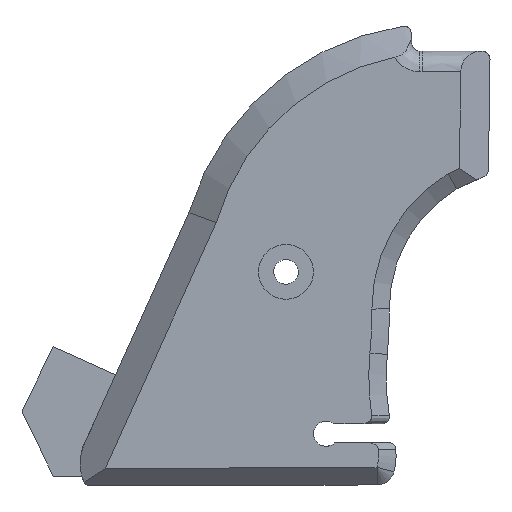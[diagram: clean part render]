
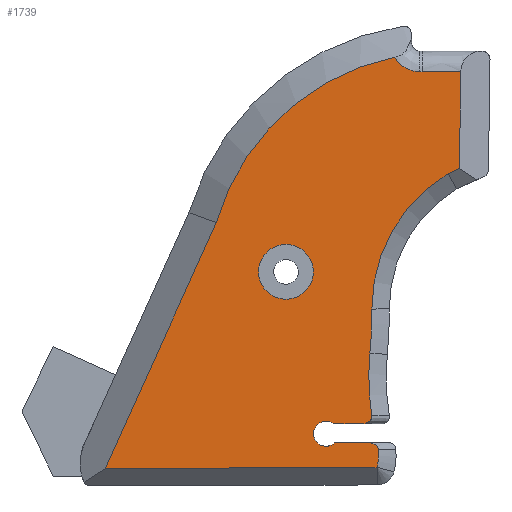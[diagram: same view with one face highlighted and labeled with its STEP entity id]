
A CAD part, left-side view. The second image highlights one B-rep face of the part: STEP entity #1739.
In plain terms, the highlighted planar face has unit normal (-1, 0, 0).
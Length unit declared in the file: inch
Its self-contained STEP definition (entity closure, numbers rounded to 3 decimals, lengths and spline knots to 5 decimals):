
#44=FACE_BOUND('',#590,.T.);
#51=PLANE('',#1873);
#114=CIRCLE('',#1874,0.08642);
#115=CIRCLE('',#1875,1.78527);
#116=CIRCLE('',#1876,3.16162);
#117=CIRCLE('',#1877,1.08448);
#118=CIRCLE('',#1878,1.6175);
#119=CIRCLE('',#1879,0.00059);
#120=CIRCLE('',#1880,0.36222);
#121=CIRCLE('',#1881,0.18906);
#183=LINE('',#2847,#329);
#184=LINE('',#2851,#330);
#185=LINE('',#2872,#331);
#186=LINE('',#2874,#332);
#187=LINE('',#2894,#333);
#188=LINE('',#2896,#334);
#329=VECTOR('',#2102,0.3937);
#330=VECTOR('',#2105,0.3937);
#331=VECTOR('',#2112,0.3937);
#332=VECTOR('',#2113,0.3937);
#333=VECTOR('',#2116,0.3937);
#334=VECTOR('',#2117,0.3937);
#490=FACE_OUTER_BOUND('',#589,.T.);
#589=EDGE_LOOP('',(#1260,#1261,#1262,#1263,#1264,#1265,#1266,#1267,#1268,
#1269,#1270,#1271,#1272,#1273,#1274,#1275,#1276,#1277));
#590=EDGE_LOOP('',(#1278));
#693=B_SPLINE_CURVE_WITH_KNOTS('',3,(#2791,#2792,#2793,#2794,#2795,#2796,
#2797,#2798,#2799,#2800),.UNSPECIFIED.,.F.,.F.,(4,2,2,2,4),(0.,0.09662,
0.17272,0.22016,0.26444),.UNSPECIFIED.);
#697=B_SPLINE_CURVE_WITH_KNOTS('',3,(#2853,#2854,#2855,#2856,#2857,#2858,
#2859,#2860,#2861,#2862,#2863,#2864),.UNSPECIFIED.,.F.,.F.,(4,2,2,2,2,4),
(0.,0.0356,0.07328,0.12123,0.18522,
0.24525),.UNSPECIFIED.);
#698=B_SPLINE_CURVE_WITH_KNOTS('',3,(#2876,#2877,#2878,#2879),
 .UNSPECIFIED.,.F.,.F.,(4,4),(-1.07364,-0.39578),
 .UNSPECIFIED.);
#699=B_SPLINE_CURVE_WITH_KNOTS('',3,(#2881,#2882,#2883,#2884),
 .UNSPECIFIED.,.F.,.F.,(4,4),(-0.04305,0.00553),
 .UNSPECIFIED.);
#700=B_SPLINE_CURVE_WITH_KNOTS('',3,(#2886,#2887,#2888,#2889,#2890),
 .UNSPECIFIED.,.F.,.F.,(4,1,4),(-0.56305,-0.47097,-0.04305),
 .UNSPECIFIED.);
#782=VERTEX_POINT('',#2785);
#783=VERTEX_POINT('',#2790);
#788=VERTEX_POINT('',#2846);
#789=VERTEX_POINT('',#2848);
#790=VERTEX_POINT('',#2850);
#791=VERTEX_POINT('',#2852);
#792=VERTEX_POINT('',#2865);
#793=VERTEX_POINT('',#2867);
#794=VERTEX_POINT('',#2869);
#795=VERTEX_POINT('',#2871);
#796=VERTEX_POINT('',#2873);
#797=VERTEX_POINT('',#2875);
#798=VERTEX_POINT('',#2880);
#799=VERTEX_POINT('',#2885);
#800=VERTEX_POINT('',#2891);
#801=VERTEX_POINT('',#2893);
#802=VERTEX_POINT('',#2895);
#803=VERTEX_POINT('',#2897);
#804=VERTEX_POINT('',#2900);
#965=EDGE_CURVE('',#782,#783,#693,.T.);
#972=EDGE_CURVE('',#782,#788,#183,.T.);
#973=EDGE_CURVE('',#788,#789,#114,.T.);
#974=EDGE_CURVE('',#789,#790,#184,.T.);
#975=EDGE_CURVE('',#791,#790,#697,.T.);
#976=EDGE_CURVE('',#792,#791,#115,.T.);
#977=EDGE_CURVE('',#793,#792,#116,.T.);
#978=EDGE_CURVE('',#794,#793,#117,.T.);
#979=EDGE_CURVE('',#795,#794,#185,.T.);
#980=EDGE_CURVE('',#796,#795,#186,.T.);
#981=EDGE_CURVE('',#797,#796,#698,.T.);
#982=EDGE_CURVE('',#798,#797,#699,.T.);
#983=EDGE_CURVE('',#799,#798,#700,.T.);
#984=EDGE_CURVE('',#800,#799,#118,.T.);
#985=EDGE_CURVE('',#801,#800,#187,.T.);
#986=EDGE_CURVE('',#802,#801,#188,.T.);
#987=EDGE_CURVE('',#803,#802,#119,.T.);
#988=EDGE_CURVE('',#783,#803,#120,.T.);
#989=EDGE_CURVE('',#804,#804,#121,.T.);
#1260=ORIENTED_EDGE('',*,*,#965,.F.);
#1261=ORIENTED_EDGE('',*,*,#972,.T.);
#1262=ORIENTED_EDGE('',*,*,#973,.T.);
#1263=ORIENTED_EDGE('',*,*,#974,.T.);
#1264=ORIENTED_EDGE('',*,*,#975,.F.);
#1265=ORIENTED_EDGE('',*,*,#976,.F.);
#1266=ORIENTED_EDGE('',*,*,#977,.F.);
#1267=ORIENTED_EDGE('',*,*,#978,.F.);
#1268=ORIENTED_EDGE('',*,*,#979,.F.);
#1269=ORIENTED_EDGE('',*,*,#980,.F.);
#1270=ORIENTED_EDGE('',*,*,#981,.F.);
#1271=ORIENTED_EDGE('',*,*,#982,.F.);
#1272=ORIENTED_EDGE('',*,*,#983,.F.);
#1273=ORIENTED_EDGE('',*,*,#984,.F.);
#1274=ORIENTED_EDGE('',*,*,#985,.F.);
#1275=ORIENTED_EDGE('',*,*,#986,.F.);
#1276=ORIENTED_EDGE('',*,*,#987,.F.);
#1277=ORIENTED_EDGE('',*,*,#988,.F.);
#1278=ORIENTED_EDGE('',*,*,#989,.T.);
#1739=ADVANCED_FACE('',(#490,#44),#51,.F.);
#1873=AXIS2_PLACEMENT_3D('',#2845,#2100,#2101);
#1874=AXIS2_PLACEMENT_3D('',#2849,#2103,#2104);
#1875=AXIS2_PLACEMENT_3D('',#2866,#2106,#2107);
#1876=AXIS2_PLACEMENT_3D('',#2868,#2108,#2109);
#1877=AXIS2_PLACEMENT_3D('',#2870,#2110,#2111);
#1878=AXIS2_PLACEMENT_3D('',#2892,#2114,#2115);
#1879=AXIS2_PLACEMENT_3D('',#2898,#2118,#2119);
#1880=AXIS2_PLACEMENT_3D('',#2899,#2120,#2121);
#1881=AXIS2_PLACEMENT_3D('',#2901,#2122,#2123);
#2100=DIRECTION('center_axis',(1.,0.,0.));
#2101=DIRECTION('ref_axis',(0.,1.,0.026));
#2102=DIRECTION('',(0.,1.,0.));
#2103=DIRECTION('center_axis',(1.,0.,0.));
#2104=DIRECTION('ref_axis',(0.,0.688,0.725));
#2105=DIRECTION('',(0.,-1.,0.));
#2106=DIRECTION('center_axis',(-1.,0.,0.));
#2107=DIRECTION('ref_axis',(0.,0.968,-0.249));
#2108=DIRECTION('center_axis',(1.,0.,0.));
#2109=DIRECTION('ref_axis',(0.,-1.,0.004));
#2110=DIRECTION('center_axis',(-1.,0.,0.));
#2111=DIRECTION('ref_axis',(0.,1.,-0.004));
#2112=DIRECTION('',(0.,0.915,-0.405));
#2113=DIRECTION('',(0.,0.014,-1.));
#2114=DIRECTION('center_axis',(1.,0.,0.));
#2115=DIRECTION('ref_axis',(0.,0.959,0.283));
#2116=DIRECTION('',(0.,-0.412,0.911));
#2117=DIRECTION('',(0.,1.,-0.003));
#2118=DIRECTION('center_axis',(1.,0.,0.));
#2119=DIRECTION('ref_axis',(0.,-0.97,-0.243));
#2120=DIRECTION('center_axis',(1.,0.,0.));
#2121=DIRECTION('ref_axis',(0.,-0.968,0.249));
#2122=DIRECTION('center_axis',(1.,0.,0.));
#2123=DIRECTION('ref_axis',(0.,-1.,0.));
#2785=CARTESIAN_POINT('',(-0.37,-2.66875,1.43));
#2790=CARTESIAN_POINT('',(-0.37,-2.73948,1.38345));
#2791=CARTESIAN_POINT('Ctrl Pts',(-0.37,-2.66875,1.43));
#2792=CARTESIAN_POINT('Ctrl Pts',(-0.37,-2.68143,1.43));
#2793=CARTESIAN_POINT('Ctrl Pts',(-0.37,-2.69387,
1.42761));
#2794=CARTESIAN_POINT('Ctrl Pts',(-0.37,-2.71339,
1.41948));
#2795=CARTESIAN_POINT('Ctrl Pts',(-0.37,-2.72078,1.41468));
#2796=CARTESIAN_POINT('Ctrl Pts',(-0.37,-2.73014,1.4054));
#2797=CARTESIAN_POINT('Ctrl Pts',(-0.37,-2.73323,1.40134));
#2798=CARTESIAN_POINT('Ctrl Pts',(-0.37,-2.73764,1.39263));
#2799=CARTESIAN_POINT('Ctrl Pts',(-0.37,-2.73902,1.38813));
#2800=CARTESIAN_POINT('Ctrl Pts',(-0.37,-2.73948,1.38345));
#2845=CARTESIAN_POINT('Origin',(-0.37,-2.10243,2.70897));
#2846=CARTESIAN_POINT('',(-0.37,-2.43902,1.43));
#2847=CARTESIAN_POINT('',(-0.37,-2.48121,1.43));
#2848=CARTESIAN_POINT('',(-0.37,-2.43174,1.56002));
#2849=CARTESIAN_POINT('Origin',(-0.37,-2.37864,1.49183));
#2850=CARTESIAN_POINT('',(-0.37,-2.62291,1.56002));
#2851=CARTESIAN_POINT('',(-0.37,-2.26708,1.56002));
#2852=CARTESIAN_POINT('',(-0.37,-2.69362,1.61534));
#2853=CARTESIAN_POINT('Ctrl Pts',(-0.37,-2.69362,1.61534));
#2854=CARTESIAN_POINT('Ctrl Pts',(-0.37,-2.69432,1.61072));
#2855=CARTESIAN_POINT('Ctrl Pts',(-0.37,-2.69411,1.60608));
#2856=CARTESIAN_POINT('Ctrl Pts',(-0.37,-2.69182,1.59674));
#2857=CARTESIAN_POINT('Ctrl Pts',(-0.37,-2.68969,1.59225));
#2858=CARTESIAN_POINT('Ctrl Pts',(-0.37,-2.68329,1.58299));
#2859=CARTESIAN_POINT('Ctrl Pts',(-0.37,-2.67866,
1.57856));
#2860=CARTESIAN_POINT('Ctrl Pts',(-0.37,-2.66663,
1.56999));
#2861=CARTESIAN_POINT('Ctrl Pts',(-0.37,-2.65841,
1.56615));
#2862=CARTESIAN_POINT('Ctrl Pts',(-0.37,-2.64076,
1.56119));
#2863=CARTESIAN_POINT('Ctrl Pts',(-0.37,-2.6318,1.56002));
#2864=CARTESIAN_POINT('Ctrl Pts',(-0.37,-2.62291,1.56002));
#2865=CARTESIAN_POINT('',(-0.37,-2.68092,2.04838));
#2866=CARTESIAN_POINT('Origin',(-0.37,-4.45858,1.88384));
#2867=CARTESIAN_POINT('',(-0.37,-2.69435,2.35087));
#2868=CARTESIAN_POINT('Origin',(-0.37,0.46725,2.33977));
#2869=CARTESIAN_POINT('',(-0.37,-3.21996,3.28407));
#2870=CARTESIAN_POINT('Origin',(-0.37,-3.77883,2.35468));
#2871=CARTESIAN_POINT('',(-0.37,-3.29722,3.31825));
#2872=CARTESIAN_POINT('',(-0.37,-2.6498,3.03182));
#2873=CARTESIAN_POINT('',(-0.37,-3.30657,3.98499));
#2874=CARTESIAN_POINT('',(-0.37,-3.29279,3.00225));
#2875=CARTESIAN_POINT('',(-0.37,-3.0397,3.98376));
#2876=CARTESIAN_POINT('Ctrl Pts',(-0.37,-3.0397,3.98376));
#2877=CARTESIAN_POINT('Ctrl Pts',(-0.37,-3.12866,3.98417));
#2878=CARTESIAN_POINT('Ctrl Pts',(-0.37,-3.21762,3.98458));
#2879=CARTESIAN_POINT('Ctrl Pts',(-0.37,-3.30657,3.98499));
#2880=CARTESIAN_POINT('',(-0.37,-3.02059,3.98426));
#2881=CARTESIAN_POINT('Ctrl Pts',(-0.37,-3.02059,3.98426));
#2882=CARTESIAN_POINT('Ctrl Pts',(-0.37,-3.02696,3.9841));
#2883=CARTESIAN_POINT('Ctrl Pts',(-0.37,-3.03333,3.98393));
#2884=CARTESIAN_POINT('Ctrl Pts',(-0.37,-3.0397,3.98376));
#2885=CARTESIAN_POINT('',(-0.37,-2.85239,4.08487));
#2886=CARTESIAN_POINT('Ctrl Pts',(-0.37,-2.85236,4.08486));
#2887=CARTESIAN_POINT('Ctrl Pts',(-0.37,-2.85834,4.07434));
#2888=CARTESIAN_POINT('Ctrl Pts',(-0.37,-2.89746,4.01804));
#2889=CARTESIAN_POINT('Ctrl Pts',(-0.37,-2.96445,3.98573));
#2890=CARTESIAN_POINT('Ctrl Pts',(-0.37,-3.02059,3.98426));
#2891=CARTESIAN_POINT('',(-0.37,-1.62343,2.94488));
#2892=CARTESIAN_POINT('Origin',(-0.37,-3.17873,2.50064));
#2893=CARTESIAN_POINT('',(-0.37,-0.85851,1.25341));
#2894=CARTESIAN_POINT('',(-0.37,-1.61687,2.93038));
#2895=CARTESIAN_POINT('',(-0.37,-2.72978,1.25969));
#2896=CARTESIAN_POINT('',(-0.37,-1.43282,1.25533));
#2897=CARTESIAN_POINT('',(-0.37,-2.73035,1.26014));
#2898=CARTESIAN_POINT('Origin',(-0.37,-2.72978,1.26028));
#2899=CARTESIAN_POINT('Origin',(-0.37,-2.37898,1.34814));
#2900=CARTESIAN_POINT('',(-0.37,-1.9138,2.60686));
#2901=CARTESIAN_POINT('Origin',(-0.37,-2.10286,2.60686));
